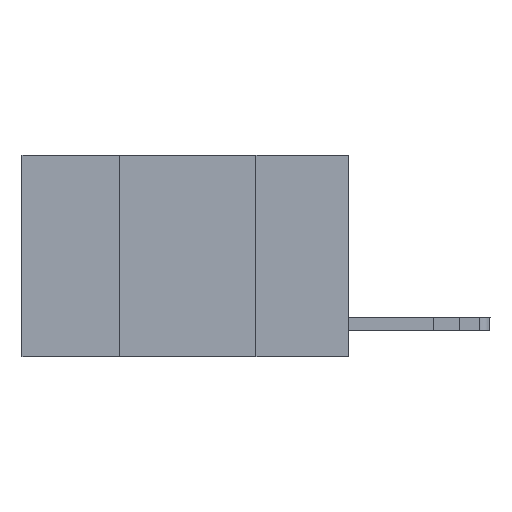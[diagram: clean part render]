
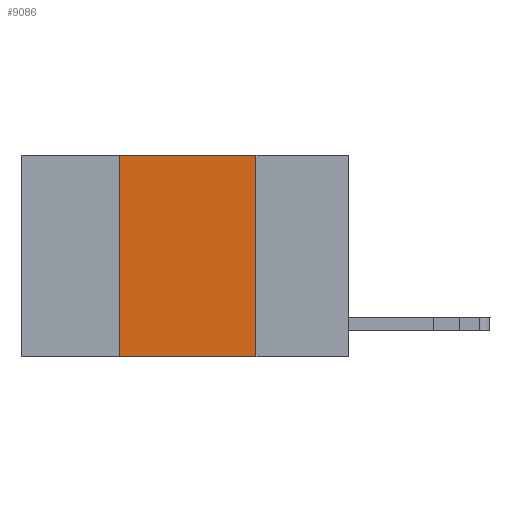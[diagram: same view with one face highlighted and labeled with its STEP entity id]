
A CAD part, left-side view. The second image highlights one B-rep face of the part: STEP entity #9086.
In plain terms, the highlighted planar face has unit normal (-1, 0, 0).
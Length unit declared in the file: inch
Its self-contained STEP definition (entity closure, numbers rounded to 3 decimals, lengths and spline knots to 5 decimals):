
#61 = DIRECTION ( 'NONE',  ( 0., 0., 1. ) ) ;
#100 = VECTOR ( 'NONE', #61, 39.37008 ) ;
#1574 = LINE ( 'NONE', #7554, #14948 ) ;
#1737 = DIRECTION ( 'NONE',  ( 0., 0., -1. ) ) ;
#2735 = AXIS2_PLACEMENT_3D ( 'NONE', #15652, #3864, #17105 ) ;
#3717 = ORIENTED_EDGE ( 'NONE', *, *, #12498, .F. ) ;
#3761 = PLANE ( 'NONE',  #2735 ) ;
#3864 = DIRECTION ( 'NONE',  ( 1., 0., 0. ) ) ;
#5957 = LINE ( 'NONE', #17921, #7459 ) ;
#6114 = ORIENTED_EDGE ( 'NONE', *, *, #6527, .F. ) ;
#6527 = EDGE_CURVE ( 'NONE', #8368, #14721, #12051, .T. ) ;
#7459 = VECTOR ( 'NONE', #1737, 39.37008 ) ;
#7554 = CARTESIAN_POINT ( 'NONE',  ( 0., 0.6, 0. ) ) ;
#7677 = CARTESIAN_POINT ( 'NONE',  ( 0., 0.42, 0. ) ) ;
#8368 = VERTEX_POINT ( 'NONE', #11073 ) ;
#8609 = ORIENTED_EDGE ( 'NONE', *, *, #11483, .F. ) ;
#9086 = ADVANCED_FACE ( 'NONE', ( #12638 ), #3761, .F. ) ;
#9758 = CARTESIAN_POINT ( 'NONE',  ( 0., 0.42, 0. ) ) ;
#9876 = CARTESIAN_POINT ( 'NONE',  ( 0., 0.17, -0.37 ) ) ;
#10468 = EDGE_LOOP ( 'NONE', ( #8609, #3717, #6114, #14292 ) ) ;
#11073 = CARTESIAN_POINT ( 'NONE',  ( 0., 0.42, -0.37 ) ) ;
#11150 = CARTESIAN_POINT ( 'NONE',  ( 0., 0.17, 0. ) ) ;
#11483 = EDGE_CURVE ( 'NONE', #19236, #14316, #5957, .T. ) ;
#12022 = DIRECTION ( 'NONE',  ( 0., -1., 0. ) ) ;
#12051 = LINE ( 'NONE', #7677, #100 ) ;
#12498 = EDGE_CURVE ( 'NONE', #14721, #19236, #1574, .T. ) ;
#12638 = FACE_OUTER_BOUND ( 'NONE', #10468, .T. ) ;
#13486 = DIRECTION ( 'NONE',  ( 0., -1., 0. ) ) ;
#13592 = CARTESIAN_POINT ( 'NONE',  ( 0., 0.6, -0.37 ) ) ;
#14292 = ORIENTED_EDGE ( 'NONE', *, *, #16676, .T. ) ;
#14316 = VERTEX_POINT ( 'NONE', #9876 ) ;
#14721 = VERTEX_POINT ( 'NONE', #9758 ) ;
#14948 = VECTOR ( 'NONE', #13486, 39.37008 ) ;
#15652 = CARTESIAN_POINT ( 'NONE',  ( 0., 0.6, 0. ) ) ;
#16251 = VECTOR ( 'NONE', #12022, 39.37008 ) ;
#16676 = EDGE_CURVE ( 'NONE', #8368, #14316, #18252, .T. ) ;
#17105 = DIRECTION ( 'NONE',  ( 0., 0., -1. ) ) ;
#17921 = CARTESIAN_POINT ( 'NONE',  ( 0., 0.17, 0. ) ) ;
#18252 = LINE ( 'NONE', #13592, #16251 ) ;
#19236 = VERTEX_POINT ( 'NONE', #11150 ) ;
